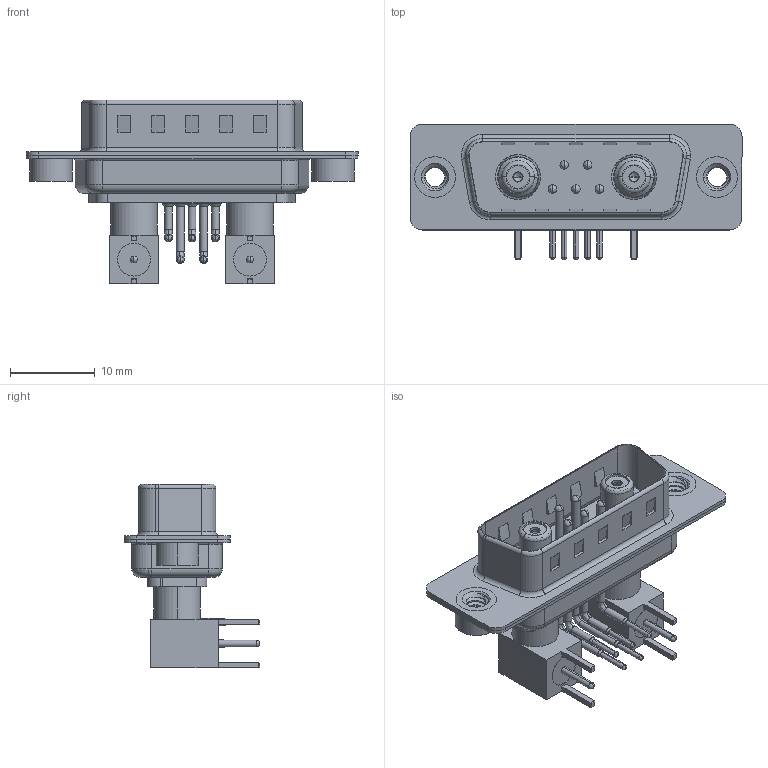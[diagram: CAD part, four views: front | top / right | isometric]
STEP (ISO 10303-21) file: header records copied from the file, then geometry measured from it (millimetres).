
FILE_DESCRIPTION (( 'STEP AP203' ), '1' );
FILE_NAME ('629-7W2-640-7TA.STEP', '2022-05-06T18:08:46', ( '' ), ( '' ), 'SwSTEP 2.0', 'SolidWorks 2020', '' );
FILE_SCHEMA (( 'CONFIG_CONTROL_DESIGN' ));
Length unit declared in the file: millimetre
Products named in the file (16): Co-Ax Jack Assy_RA; 629Combo Contact Row 1; 629Combo Shell Front_15 Contacts; Insulator RA Pin; Insulator Socket 2; 629Combo Threaded Rivet_2; Insulator Socket; 629Combo Housing_7W2; Socket_RA; 629Combo Shell Rear_15 Contacts; Co-Ax Jack_RA PC Tail; 629-7W2-640-7TA; RA Back Shell; Locking Collar; 629Combo Contact Row 2
Assembly tree (26 placements, depth 3):
  629-7W2-640-7TA
    629Combo Housing_7W2
    629Combo Shell Rear_15 Contacts
    629Combo Shell Front_15 Contacts
    629Combo Threaded Rivet_2  x2
    Co-Ax Jack Assy_RA
      Co-Ax Jack_RA PC Tail
      Insulator Socket
      Insulator Socket 2
      Locking Collar
      Socket_RA
      RA Back Shell
      Insulator RA Pin
    Co-Ax Jack Assy_RA
      Co-Ax Jack_RA PC Tail
      Insulator Socket
      Insulator Socket 2
      Locking Collar
      Socket_RA
      RA Back Shell
      Insulator RA Pin
    629Combo Contact Row 1  x2
    629Combo Contact Row 2  x3
Bounding box: 39.2 x 16 x 21.71 mm (x, y, z)
Volume: 2451.7 mm3; surface area: 6783.3 mm2
Topology: 24 solids, 24 shells, 1194 faces, 3101 edges, 1978 vertices
Faces by surface type: plane 573, cylinder 447, cone 70, torus 62, bspline 38, sphere 4
Entity records: 25170 total; most frequent: CARTESIAN_POINT 5584, DIRECTION 3830, ORIENTED_EDGE 3578, EDGE_CURVE 1789, AXIS2_PLACEMENT_3D 1383, VERTEX_POINT 1147, LINE 1064, VECTOR 1064
